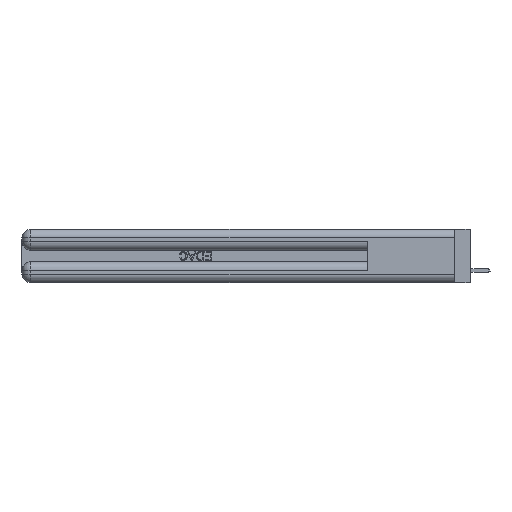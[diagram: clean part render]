
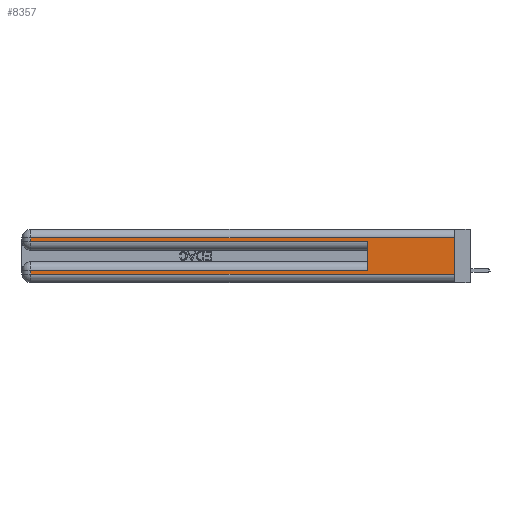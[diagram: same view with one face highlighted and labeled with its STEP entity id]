
A CAD part, left-side view. The second image highlights one B-rep face of the part: STEP entity #8357.
In plain terms, the highlighted planar face has unit normal (-1, 0, 0).
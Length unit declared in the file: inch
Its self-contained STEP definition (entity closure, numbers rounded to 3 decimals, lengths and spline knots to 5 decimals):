
#17 = ORIENTED_EDGE ( 'NONE', *, *, #24729, .T. ) ;
#372 = VERTEX_POINT ( 'NONE', #16597 ) ;
#1567 = LINE ( 'NONE', #24178, #3362 ) ;
#1872 = DIRECTION ( 'NONE',  ( 1., 0., 0. ) ) ;
#2707 = VECTOR ( 'NONE', #46338, 39.37008 ) ;
#2794 = EDGE_CURVE ( 'NONE', #9082, #43722, #23163, .T. ) ;
#2967 = ORIENTED_EDGE ( 'NONE', *, *, #2794, .F. ) ;
#3362 = VECTOR ( 'NONE', #5662, 39.37008 ) ;
#4240 = EDGE_LOOP ( 'NONE', ( #12704, #42405, #17, #21442, #2967, #45321, #12779, #6761 ) ) ;
#4620 = CARTESIAN_POINT ( 'NONE',  ( 0., 2.94, 0.085 ) ) ;
#5175 = VERTEX_POINT ( 'NONE', #28078 ) ;
#5662 = DIRECTION ( 'NONE',  ( 0., 1., 0. ) ) ;
#6761 = ORIENTED_EDGE ( 'NONE', *, *, #43045, .T. ) ;
#7367 = EDGE_CURVE ( 'NONE', #9082, #46248, #9129, .T. ) ;
#7914 = AXIS2_PLACEMENT_3D ( 'NONE', #23935, #1872, #19688 ) ;
#8090 = EDGE_CURVE ( 'NONE', #34157, #372, #21150, .T. ) ;
#8357 = ADVANCED_FACE ( 'NONE', ( #17059 ), #16330, .F. ) ;
#8955 = CARTESIAN_POINT ( 'NONE',  ( 0., 0.6, 0.085 ) ) ;
#9082 = VERTEX_POINT ( 'NONE', #8955 ) ;
#9129 = LINE ( 'NONE', #12017, #45799 ) ;
#12017 = CARTESIAN_POINT ( 'NONE',  ( 0., 0., 0.085 ) ) ;
#12596 = CARTESIAN_POINT ( 'NONE',  ( 0., 0., 0.31 ) ) ;
#12704 = ORIENTED_EDGE ( 'NONE', *, *, #8090, .F. ) ;
#12779 = ORIENTED_EDGE ( 'NONE', *, *, #21415, .T. ) ;
#16330 = PLANE ( 'NONE',  #7914 ) ;
#16468 = CARTESIAN_POINT ( 'NONE',  ( 0., 2.94, 0.31 ) ) ;
#16597 = CARTESIAN_POINT ( 'NONE',  ( 0., 0., 0.06 ) ) ;
#16693 = VECTOR ( 'NONE', #34717, 39.37008 ) ;
#17059 = FACE_OUTER_BOUND ( 'NONE', #4240, .T. ) ;
#19683 = DIRECTION ( 'NONE',  ( 0., -1., 0. ) ) ;
#19688 = DIRECTION ( 'NONE',  ( 0., 0., -1. ) ) ;
#19987 = CARTESIAN_POINT ( 'NONE',  ( 0., 2.94, 0.37 ) ) ;
#20599 = CARTESIAN_POINT ( 'NONE',  ( 0., 0., 0.06 ) ) ;
#21121 = LINE ( 'NONE', #20599, #2707 ) ;
#21150 = LINE ( 'NONE', #34668, #30262 ) ;
#21395 = VERTEX_POINT ( 'NONE', #16468 ) ;
#21415 = EDGE_CURVE ( 'NONE', #46248, #5175, #46533, .T. ) ;
#21442 = ORIENTED_EDGE ( 'NONE', *, *, #33587, .T. ) ;
#22681 = EDGE_CURVE ( 'NONE', #34157, #21395, #1567, .T. ) ;
#23079 = CARTESIAN_POINT ( 'NONE',  ( 0., 2.94, 0.37 ) ) ;
#23163 = LINE ( 'NONE', #33255, #44337 ) ;
#23199 = DIRECTION ( 'NONE',  ( 0., 1., 0. ) ) ;
#23935 = CARTESIAN_POINT ( 'NONE',  ( 0., 0., 0.37 ) ) ;
#24178 = CARTESIAN_POINT ( 'NONE',  ( 0., 0., 0.31 ) ) ;
#24729 = EDGE_CURVE ( 'NONE', #21395, #34283, #26104, .T. ) ;
#26104 = LINE ( 'NONE', #23079, #36410 ) ;
#26942 = CARTESIAN_POINT ( 'NONE',  ( 0., 0., 0.285 ) ) ;
#27631 = CARTESIAN_POINT ( 'NONE',  ( 0., 2.94, 0.285 ) ) ;
#28078 = CARTESIAN_POINT ( 'NONE',  ( 0., 2.94, 0.06 ) ) ;
#28580 = CARTESIAN_POINT ( 'NONE',  ( 0., 0.6, 0.285 ) ) ;
#30262 = VECTOR ( 'NONE', #45404, 39.37008 ) ;
#30431 = DIRECTION ( 'NONE',  ( 0., 0., -1. ) ) ;
#32567 = LINE ( 'NONE', #26942, #33633 ) ;
#33255 = CARTESIAN_POINT ( 'NONE',  ( 0., 0.6, 0.145 ) ) ;
#33587 = EDGE_CURVE ( 'NONE', #34283, #43722, #32567, .T. ) ;
#33633 = VECTOR ( 'NONE', #19683, 39.37008 ) ;
#34157 = VERTEX_POINT ( 'NONE', #12596 ) ;
#34283 = VERTEX_POINT ( 'NONE', #27631 ) ;
#34668 = CARTESIAN_POINT ( 'NONE',  ( 0., 0., 0.37 ) ) ;
#34717 = DIRECTION ( 'NONE',  ( 0., 0., -1. ) ) ;
#36410 = VECTOR ( 'NONE', #30431, 39.37008 ) ;
#40744 = DIRECTION ( 'NONE',  ( 0., 0., 1. ) ) ;
#42405 = ORIENTED_EDGE ( 'NONE', *, *, #22681, .T. ) ;
#43045 = EDGE_CURVE ( 'NONE', #5175, #372, #21121, .T. ) ;
#43722 = VERTEX_POINT ( 'NONE', #28580 ) ;
#44337 = VECTOR ( 'NONE', #40744, 39.37008 ) ;
#45321 = ORIENTED_EDGE ( 'NONE', *, *, #7367, .T. ) ;
#45404 = DIRECTION ( 'NONE',  ( 0., 0., -1. ) ) ;
#45799 = VECTOR ( 'NONE', #23199, 39.37008 ) ;
#46248 = VERTEX_POINT ( 'NONE', #4620 ) ;
#46338 = DIRECTION ( 'NONE',  ( 0., -1., 0. ) ) ;
#46533 = LINE ( 'NONE', #19987, #16693 ) ;
